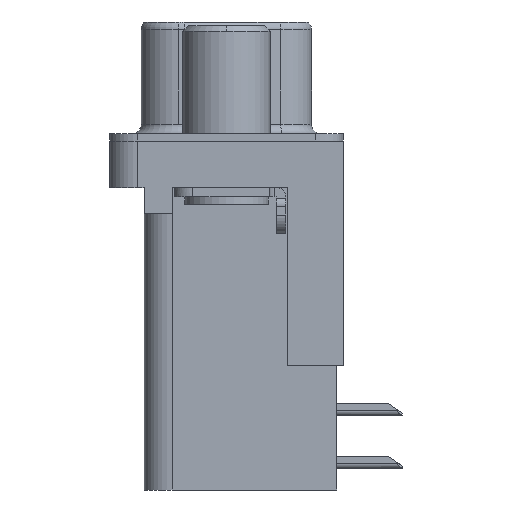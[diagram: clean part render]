
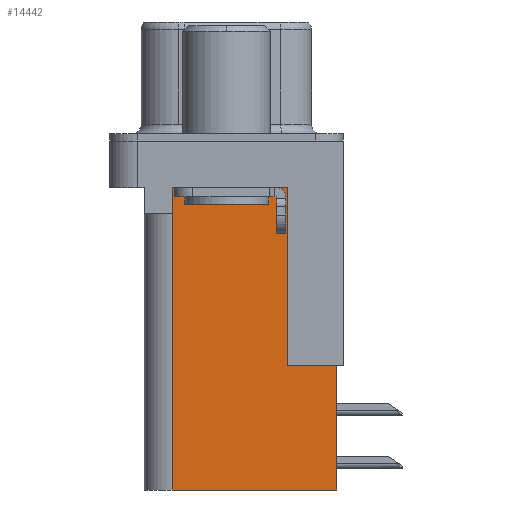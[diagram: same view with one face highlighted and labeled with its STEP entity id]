
A CAD part, left-side view. The second image highlights one B-rep face of the part: STEP entity #14442.
In plain terms, the highlighted planar face has unit normal (-1, 0, 0).
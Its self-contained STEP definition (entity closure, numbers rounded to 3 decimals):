
#17 = VECTOR ( 'NONE', #17790, 1000. ) ;
#91 = LINE ( 'NONE', #15088, #17 ) ;
#469 = CARTESIAN_POINT ( 'NONE',  ( 3.765, -5.925, -12.05 ) ) ;
#909 = CARTESIAN_POINT ( 'NONE',  ( 3.765, 2.895, -3.9 ) ) ;
#1015 = VERTEX_POINT ( 'NONE', #13812 ) ;
#1141 = PLANE ( 'NONE',  #15176 ) ;
#1616 = CARTESIAN_POINT ( 'NONE',  ( 3.765, -5.925, -18.76 ) ) ;
#1624 = CARTESIAN_POINT ( 'NONE',  ( 3.765, -6.295, -12.05 ) ) ;
#2206 = ORIENTED_EDGE ( 'NONE', *, *, #4745, .T. ) ;
#2271 = CARTESIAN_POINT ( 'NONE',  ( 3.765, -3.295, -18.76 ) ) ;
#2337 = ORIENTED_EDGE ( 'NONE', *, *, #8556, .T. ) ;
#2506 = DIRECTION ( 'NONE',  ( 0., 1., 0. ) ) ;
#2569 = EDGE_CURVE ( 'NONE', #5281, #1015, #8937, .T. ) ;
#2715 = DIRECTION ( 'NONE',  ( 0., 1., 0. ) ) ;
#2756 = VECTOR ( 'NONE', #18995, 1000. ) ;
#2826 = LINE ( 'NONE', #4808, #2756 ) ;
#3180 = VERTEX_POINT ( 'NONE', #469 ) ;
#3284 = VECTOR ( 'NONE', #18704, 1000. ) ;
#3329 = LINE ( 'NONE', #14253, #3284 ) ;
#3435 = ORIENTED_EDGE ( 'NONE', *, *, #2569, .T. ) ;
#4215 = VECTOR ( 'NONE', #12631, 1000. ) ;
#4220 = ORIENTED_EDGE ( 'NONE', *, *, #9022, .T. ) ;
#4240 = LINE ( 'NONE', #18527, #4215 ) ;
#4601 = VERTEX_POINT ( 'NONE', #909 ) ;
#4745 = EDGE_CURVE ( 'NONE', #1015, #7521, #2826, .T. ) ;
#4808 = CARTESIAN_POINT ( 'NONE',  ( 3.765, -3.295, -2.5 ) ) ;
#5281 = VERTEX_POINT ( 'NONE', #9317 ) ;
#5299 = LINE ( 'NONE', #1624, #5314 ) ;
#5314 = VECTOR ( 'NONE', #2506, 1000. ) ;
#5516 = EDGE_CURVE ( 'NONE', #16491, #17609, #91, .T. ) ;
#5955 = VERTEX_POINT ( 'NONE', #8812 ) ;
#6494 = EDGE_CURVE ( 'NONE', #7521, #4601, #13640, .T. ) ;
#7521 = VERTEX_POINT ( 'NONE', #9141 ) ;
#7820 = ORIENTED_EDGE ( 'NONE', *, *, #16288, .F. ) ;
#8028 = DIRECTION ( 'NONE',  ( 0., 0., -1. ) ) ;
#8042 = DIRECTION ( 'NONE',  ( 0., 0., -1. ) ) ;
#8227 = VECTOR ( 'NONE', #8028, 1000. ) ;
#8369 = LINE ( 'NONE', #13331, #8227 ) ;
#8556 = EDGE_CURVE ( 'NONE', #3180, #5281, #5299, .T. ) ;
#8812 = CARTESIAN_POINT ( 'NONE',  ( 3.765, 2.925, -3.9 ) ) ;
#8875 = FACE_OUTER_BOUND ( 'NONE', #9431, .T. ) ;
#8883 = VECTOR ( 'NONE', #13773, 1000. ) ;
#8937 = LINE ( 'NONE', #2271, #8883 ) ;
#9022 = EDGE_CURVE ( 'NONE', #4601, #5955, #3329, .T. ) ;
#9141 = CARTESIAN_POINT ( 'NONE',  ( 3.765, 2.895, -2.5 ) ) ;
#9176 = CARTESIAN_POINT ( 'NONE',  ( 3.765, 2.895, -3.9 ) ) ;
#9317 = CARTESIAN_POINT ( 'NONE',  ( 3.765, -3.295, -12.05 ) ) ;
#9431 = EDGE_LOOP ( 'NONE', ( #2206, #10828, #4220, #7820, #17128, #10580, #2337, #3435 ) ) ;
#10580 = ORIENTED_EDGE ( 'NONE', *, *, #14714, .F. ) ;
#10828 = ORIENTED_EDGE ( 'NONE', *, *, #6494, .T. ) ;
#11473 = DIRECTION ( 'NONE',  ( 1., 0., 0. ) ) ;
#12631 = DIRECTION ( 'NONE',  ( 0., 0., 1. ) ) ;
#12657 = CARTESIAN_POINT ( 'NONE',  ( 3.765, 2.925, -18.76 ) ) ;
#13331 = CARTESIAN_POINT ( 'NONE',  ( 3.765, -5.925, -2. ) ) ;
#13602 = VECTOR ( 'NONE', #8042, 1000. ) ;
#13640 = LINE ( 'NONE', #9176, #13602 ) ;
#13773 = DIRECTION ( 'NONE',  ( 0., 0., 1. ) ) ;
#13812 = CARTESIAN_POINT ( 'NONE',  ( 3.765, -3.295, -2.5 ) ) ;
#14253 = CARTESIAN_POINT ( 'NONE',  ( 3.765, 0., -3.9 ) ) ;
#14442 = ADVANCED_FACE ( 'NONE', ( #8875 ), #1141, .F. ) ;
#14714 = EDGE_CURVE ( 'NONE', #3180, #16491, #8369, .T. ) ;
#15088 = CARTESIAN_POINT ( 'NONE',  ( 3.765, -3.295, -18.76 ) ) ;
#15176 = AXIS2_PLACEMENT_3D ( 'NONE', #17259, #11473, #2715 ) ;
#16288 = EDGE_CURVE ( 'NONE', #17609, #5955, #4240, .T. ) ;
#16491 = VERTEX_POINT ( 'NONE', #1616 ) ;
#17128 = ORIENTED_EDGE ( 'NONE', *, *, #5516, .F. ) ;
#17259 = CARTESIAN_POINT ( 'NONE',  ( 3.765, -3.295, -18.76 ) ) ;
#17609 = VERTEX_POINT ( 'NONE', #12657 ) ;
#17790 = DIRECTION ( 'NONE',  ( 0., 1., 0. ) ) ;
#18527 = CARTESIAN_POINT ( 'NONE',  ( 3.765, 2.925, -18.76 ) ) ;
#18704 = DIRECTION ( 'NONE',  ( 0., 1., 0. ) ) ;
#18995 = DIRECTION ( 'NONE',  ( 0., 1., 0. ) ) ;
